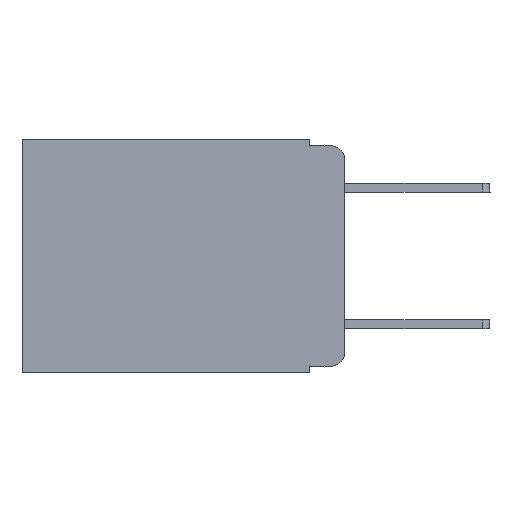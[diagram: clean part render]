
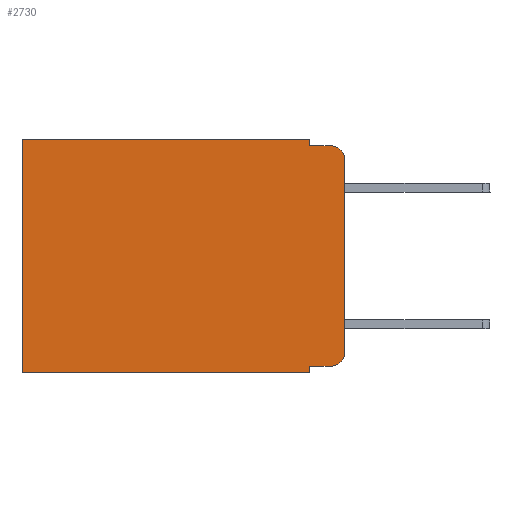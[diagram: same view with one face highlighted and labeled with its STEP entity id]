
A CAD part, left-side view. The second image highlights one B-rep face of the part: STEP entity #2730.
In plain terms, the highlighted planar face has unit normal (-1, 0, 0).
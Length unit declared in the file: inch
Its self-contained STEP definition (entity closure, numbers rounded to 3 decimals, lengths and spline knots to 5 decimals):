
#32 = CARTESIAN_POINT ( 'NONE',  ( 0.298, 0.02, -0.333 ) ) ;
#313 = LINE ( 'NONE', #4008, #3458 ) ;
#500 = EDGE_CURVE ( 'NONE', #8913, #9750, #5276, .T. ) ;
#788 = VECTOR ( 'NONE', #6280, 39.37008 ) ;
#965 = VERTEX_POINT ( 'NONE', #32 ) ;
#1064 = LINE ( 'NONE', #3556, #788 ) ;
#1589 = AXIS2_PLACEMENT_3D ( 'NONE', #8178, #1889, #1770 ) ;
#1764 = VERTEX_POINT ( 'NONE', #4673 ) ;
#1770 = DIRECTION ( 'NONE',  ( 0., 0., -1. ) ) ;
#1889 = DIRECTION ( 'NONE',  ( -1., 0., 0. ) ) ;
#2063 = CARTESIAN_POINT ( 'NONE',  ( 0.298, 0.02, -0.01 ) ) ;
#2115 = VERTEX_POINT ( 'NONE', #4825 ) ;
#2263 = CARTESIAN_POINT ( 'NONE',  ( 0.298, 0.051, -0.343 ) ) ;
#2386 = LINE ( 'NONE', #9567, #9372 ) ;
#2730 = ADVANCED_FACE ( 'NONE', ( #4374 ), #6320, .F. ) ;
#2818 = CARTESIAN_POINT ( 'NONE',  ( 0.298, 0.051, -0.333 ) ) ;
#3161 = VERTEX_POINT ( 'NONE', #11604 ) ;
#3399 = ORIENTED_EDGE ( 'NONE', *, *, #9383, .F. ) ;
#3458 = VECTOR ( 'NONE', #7700, 39.37008 ) ;
#3556 = CARTESIAN_POINT ( 'NONE',  ( 0.298, 0., 0. ) ) ;
#3680 = CIRCLE ( 'NONE', #1589, 0.02 ) ;
#4008 = CARTESIAN_POINT ( 'NONE',  ( 0.298, 0.051, -0.01 ) ) ;
#4119 = ORIENTED_EDGE ( 'NONE', *, *, #4519, .T. ) ;
#4297 = DIRECTION ( 'NONE',  ( 0., -1., 0. ) ) ;
#4374 = FACE_OUTER_BOUND ( 'NONE', #10907, .T. ) ;
#4519 = EDGE_CURVE ( 'NONE', #8913, #965, #6133, .T. ) ;
#4673 = CARTESIAN_POINT ( 'NONE',  ( 0.298, 0., -0.313 ) ) ;
#4754 = ORIENTED_EDGE ( 'NONE', *, *, #9743, .T. ) ;
#4825 = CARTESIAN_POINT ( 'NONE',  ( 0.298, 0., -0.03 ) ) ;
#4827 = EDGE_CURVE ( 'NONE', #2115, #1764, #11343, .T. ) ;
#4895 = DIRECTION ( 'NONE',  ( 0., 0., -1. ) ) ;
#5220 = VERTEX_POINT ( 'NONE', #8421 ) ;
#5229 = VECTOR ( 'NONE', #5383, 39.37008 ) ;
#5243 = CARTESIAN_POINT ( 'NONE',  ( 0.298, 0.051, -0.01 ) ) ;
#5276 = LINE ( 'NONE', #8884, #11734 ) ;
#5383 = DIRECTION ( 'NONE',  ( 0., 1., 0. ) ) ;
#5477 = ORIENTED_EDGE ( 'NONE', *, *, #8046, .F. ) ;
#5576 = EDGE_CURVE ( 'NONE', #10202, #3161, #1064, .T. ) ;
#5667 = EDGE_CURVE ( 'NONE', #10028, #7409, #313, .T. ) ;
#5773 = DIRECTION ( 'NONE',  ( -1., 0., 0. ) ) ;
#6133 = LINE ( 'NONE', #9691, #6660 ) ;
#6280 = DIRECTION ( 'NONE',  ( 0., 1., 0. ) ) ;
#6320 = PLANE ( 'NONE',  #9837 ) ;
#6660 = VECTOR ( 'NONE', #4297, 39.37008 ) ;
#7026 = DIRECTION ( 'NONE',  ( 0., 0., -1. ) ) ;
#7084 = DIRECTION ( 'NONE',  ( 0., 0., -1. ) ) ;
#7194 = EDGE_CURVE ( 'NONE', #2115, #7409, #3680, .T. ) ;
#7303 = CIRCLE ( 'NONE', #10525, 0.02 ) ;
#7409 = VERTEX_POINT ( 'NONE', #2063 ) ;
#7531 = ORIENTED_EDGE ( 'NONE', *, *, #5667, .F. ) ;
#7657 = CARTESIAN_POINT ( 'NONE',  ( 0.298, 0., 0. ) ) ;
#7700 = DIRECTION ( 'NONE',  ( 0., -1., 0. ) ) ;
#7863 = ORIENTED_EDGE ( 'NONE', *, *, #7194, .T. ) ;
#7899 = ORIENTED_EDGE ( 'NONE', *, *, #8267, .T. ) ;
#7913 = ORIENTED_EDGE ( 'NONE', *, *, #4827, .F. ) ;
#7986 = CARTESIAN_POINT ( 'NONE',  ( 0.298, 0., 0. ) ) ;
#8016 = ORIENTED_EDGE ( 'NONE', *, *, #5576, .T. ) ;
#8046 = EDGE_CURVE ( 'NONE', #10202, #10028, #11672, .T. ) ;
#8178 = CARTESIAN_POINT ( 'NONE',  ( 0.298, 0.02, -0.03 ) ) ;
#8267 = EDGE_CURVE ( 'NONE', #965, #1764, #7303, .T. ) ;
#8421 = CARTESIAN_POINT ( 'NONE',  ( 0.298, 0.473, -0.343 ) ) ;
#8436 = CARTESIAN_POINT ( 'NONE',  ( 0.298, 0.02, -0.313 ) ) ;
#8821 = VECTOR ( 'NONE', #10883, 39.37008 ) ;
#8865 = DIRECTION ( 'NONE',  ( 0., 0., -1. ) ) ;
#8884 = CARTESIAN_POINT ( 'NONE',  ( 0.298, 0.051, 0. ) ) ;
#8912 = CARTESIAN_POINT ( 'NONE',  ( 0.298, 0.051, 0. ) ) ;
#8913 = VERTEX_POINT ( 'NONE', #2818 ) ;
#9053 = CARTESIAN_POINT ( 'NONE',  ( 0.298, 0.051, 0. ) ) ;
#9372 = VECTOR ( 'NONE', #8865, 39.37008 ) ;
#9383 = EDGE_CURVE ( 'NONE', #9750, #5220, #10105, .T. ) ;
#9388 = DIRECTION ( 'NONE',  ( 0., 0., -1. ) ) ;
#9567 = CARTESIAN_POINT ( 'NONE',  ( 0.298, 0.473, 0. ) ) ;
#9691 = CARTESIAN_POINT ( 'NONE',  ( 0.298, 0.051, -0.333 ) ) ;
#9743 = EDGE_CURVE ( 'NONE', #3161, #5220, #2386, .T. ) ;
#9750 = VERTEX_POINT ( 'NONE', #2263 ) ;
#9837 = AXIS2_PLACEMENT_3D ( 'NONE', #7986, #11561, #7026 ) ;
#9999 = CARTESIAN_POINT ( 'NONE',  ( 0.298, 0., -0.343 ) ) ;
#10028 = VERTEX_POINT ( 'NONE', #5243 ) ;
#10105 = LINE ( 'NONE', #9999, #5229 ) ;
#10202 = VERTEX_POINT ( 'NONE', #8912 ) ;
#10525 = AXIS2_PLACEMENT_3D ( 'NONE', #8436, #5773, #9388 ) ;
#10883 = DIRECTION ( 'NONE',  ( 0., 0., -1. ) ) ;
#10907 = EDGE_LOOP ( 'NONE', ( #7913, #7863, #7531, #5477, #8016, #4754, #3399, #11669, #4119, #7899 ) ) ;
#11212 = VECTOR ( 'NONE', #4895, 39.37008 ) ;
#11343 = LINE ( 'NONE', #7657, #11212 ) ;
#11561 = DIRECTION ( 'NONE',  ( 1., 0., 0. ) ) ;
#11604 = CARTESIAN_POINT ( 'NONE',  ( 0.298, 0.473, 0. ) ) ;
#11669 = ORIENTED_EDGE ( 'NONE', *, *, #500, .F. ) ;
#11672 = LINE ( 'NONE', #9053, #8821 ) ;
#11734 = VECTOR ( 'NONE', #7084, 39.37008 ) ;
